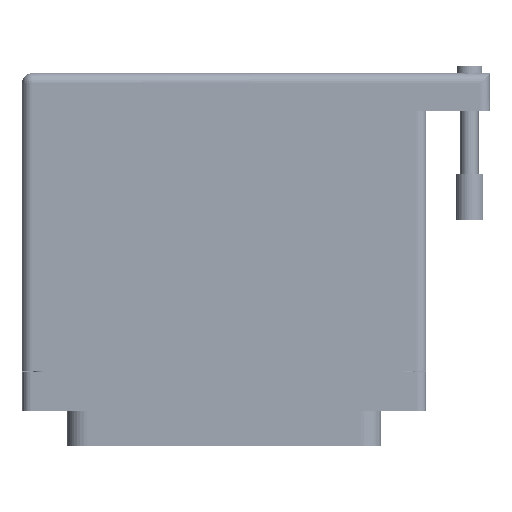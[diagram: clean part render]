
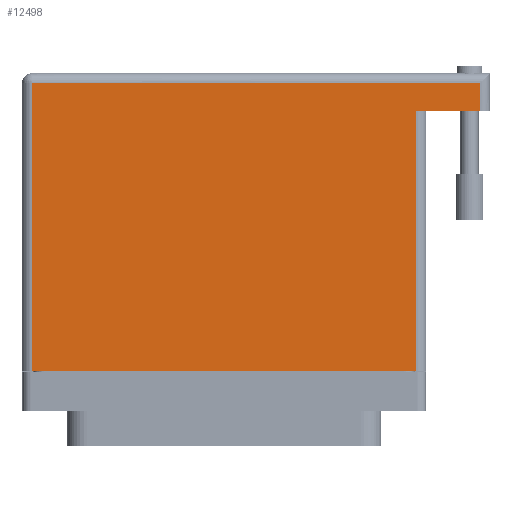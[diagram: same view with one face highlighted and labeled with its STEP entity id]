
A CAD part, front view. The second image highlights one B-rep face of the part: STEP entity #12498.
In plain terms, the highlighted face is planar.
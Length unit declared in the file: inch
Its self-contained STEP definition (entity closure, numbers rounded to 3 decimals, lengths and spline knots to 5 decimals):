
#233 = DIRECTION ( 'NONE',  ( 0., 1., 0. ) ) ;
#1325 = DIRECTION ( 'NONE',  ( 0., -1., 0. ) ) ;
#1419 = ORIENTED_EDGE ( 'NONE', *, *, #49120, .T. ) ;
#1800 = VERTEX_POINT ( 'NONE', #58872 ) ;
#3594 = VECTOR ( 'NONE', #233, 39.37008 ) ;
#3699 = LINE ( 'NONE', #74984, #23851 ) ;
#5219 = DIRECTION ( 'NONE',  ( -1., 0., 0. ) ) ;
#6483 = EDGE_CURVE ( 'NONE', #70564, #37437, #39525, .T. ) ;
#9852 = ORIENTED_EDGE ( 'NONE', *, *, #22417, .T. ) ;
#11840 = ORIENTED_EDGE ( 'NONE', *, *, #44225, .T. ) ;
#12498 = ADVANCED_FACE ( 'NONE', ( #87424 ), #12766, .F. ) ;
#12766 = PLANE ( 'NONE',  #17998 ) ;
#15891 = ORIENTED_EDGE ( 'NONE', *, *, #34250, .F. ) ;
#16686 = DIRECTION ( 'NONE',  ( 0., 1., 0. ) ) ;
#17993 = EDGE_CURVE ( 'NONE', #19664, #1800, #91875, .T. ) ;
#17998 = AXIS2_PLACEMENT_3D ( 'NONE', #84994, #84350, #5219 ) ;
#19664 = VERTEX_POINT ( 'NONE', #81101 ) ;
#22417 = EDGE_CURVE ( 'NONE', #37437, #54175, #80918, .T. ) ;
#23354 = CARTESIAN_POINT ( 'NONE',  ( -1.3775, 1.86, 0.765 ) ) ;
#23851 = VECTOR ( 'NONE', #45658, 39.37008 ) ;
#29328 = CARTESIAN_POINT ( 'NONE',  ( 1.7425, 1.86, 0.765 ) ) ;
#29551 = VECTOR ( 'NONE', #1325, 39.37008 ) ;
#29909 = LINE ( 'NONE', #80164, #33239 ) ;
#31731 = CARTESIAN_POINT ( 'NONE',  ( -1.3075, 1.86, 0.765 ) ) ;
#33239 = VECTOR ( 'NONE', #16686, 39.37008 ) ;
#33648 = VECTOR ( 'NONE', #91413, 39.37008 ) ;
#34069 = VERTEX_POINT ( 'NONE', #48296 ) ;
#34250 = EDGE_CURVE ( 'NONE', #70564, #34069, #3699, .T. ) ;
#36262 = CARTESIAN_POINT ( 'NONE',  ( 1.7425, 1.93, 0.765 ) ) ;
#37431 = LINE ( 'NONE', #51992, #29551 ) ;
#37437 = VERTEX_POINT ( 'NONE', #29328 ) ;
#39525 = LINE ( 'NONE', #36262, #3594 ) ;
#40044 = ORIENTED_EDGE ( 'NONE', *, *, #17993, .T. ) ;
#44225 = EDGE_CURVE ( 'NONE', #1800, #34069, #29909, .T. ) ;
#45658 = DIRECTION ( 'NONE',  ( -1., 0., 0. ) ) ;
#48296 = CARTESIAN_POINT ( 'NONE',  ( 1.3075, 1.674, 0.765 ) ) ;
#49120 = EDGE_CURVE ( 'NONE', #54175, #19664, #37431, .T. ) ;
#51992 = CARTESIAN_POINT ( 'NONE',  ( -1.3075, -0.1, 0.765 ) ) ;
#54175 = VERTEX_POINT ( 'NONE', #31731 ) ;
#56349 = CARTESIAN_POINT ( 'NONE',  ( -1.3775, -0.1, 0.765 ) ) ;
#58872 = CARTESIAN_POINT ( 'NONE',  ( 1.3075, -0.1, 0.765 ) ) ;
#64194 = VECTOR ( 'NONE', #88396, 39.37008 ) ;
#70564 = VERTEX_POINT ( 'NONE', #82575 ) ;
#74984 = CARTESIAN_POINT ( 'NONE',  ( 1.8125, 1.674, 0.765 ) ) ;
#79722 = ORIENTED_EDGE ( 'NONE', *, *, #6483, .T. ) ;
#80164 = CARTESIAN_POINT ( 'NONE',  ( 1.3075, 1.674, 0.765 ) ) ;
#80918 = LINE ( 'NONE', #23354, #64194 ) ;
#81101 = CARTESIAN_POINT ( 'NONE',  ( -1.3075, -0.1, 0.765 ) ) ;
#82575 = CARTESIAN_POINT ( 'NONE',  ( 1.7425, 1.674, 0.765 ) ) ;
#84350 = DIRECTION ( 'NONE',  ( 0., 0., -1. ) ) ;
#84994 = CARTESIAN_POINT ( 'NONE',  ( -1.3775, 1.93, 0.765 ) ) ;
#87424 = FACE_OUTER_BOUND ( 'NONE', #92144, .T. ) ;
#88396 = DIRECTION ( 'NONE',  ( -1., 0., 0. ) ) ;
#91413 = DIRECTION ( 'NONE',  ( 1., 0., 0. ) ) ;
#91875 = LINE ( 'NONE', #56349, #33648 ) ;
#92144 = EDGE_LOOP ( 'NONE', ( #40044, #11840, #15891, #79722, #9852, #1419 ) ) ;
